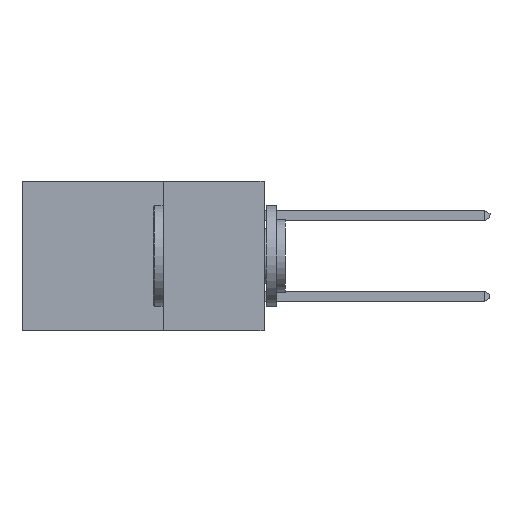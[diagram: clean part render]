
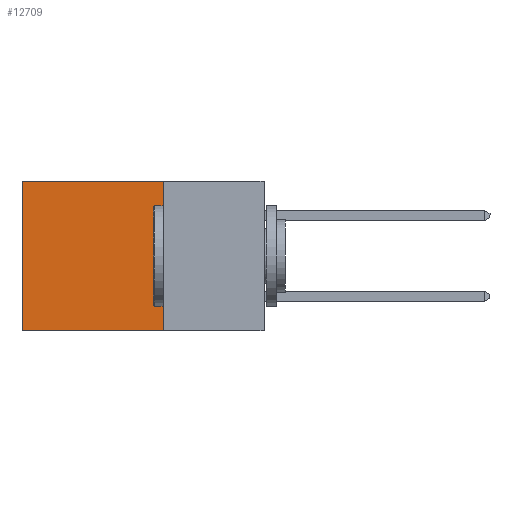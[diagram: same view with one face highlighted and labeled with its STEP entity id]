
A CAD part, left-side view. The second image highlights one B-rep face of the part: STEP entity #12709.
In plain terms, the highlighted planar face has unit normal (-1, 0, 0).
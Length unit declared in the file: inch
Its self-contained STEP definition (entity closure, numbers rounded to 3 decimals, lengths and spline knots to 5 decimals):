
#444 = DIRECTION ( 'NONE',  ( 0., 1., 0. ) ) ;
#577 = ORIENTED_EDGE ( 'NONE', *, *, #9181, .T. ) ;
#768 = VERTEX_POINT ( 'NONE', #5218 ) ;
#2378 = AXIS2_PLACEMENT_3D ( 'NONE', #11979, #4411, #13243 ) ;
#2916 = LINE ( 'NONE', #13124, #12667 ) ;
#3073 = PLANE ( 'NONE',  #2378 ) ;
#4386 = VECTOR ( 'NONE', #13675, 39.37008 ) ;
#4411 = DIRECTION ( 'NONE',  ( 1., 0., 0. ) ) ;
#4799 = LINE ( 'NONE', #8060, #4386 ) ;
#4808 = EDGE_CURVE ( 'NONE', #10295, #5547, #4799, .T. ) ;
#5218 = CARTESIAN_POINT ( 'NONE',  ( 0.298, 0.6, -0.37 ) ) ;
#5322 = DIRECTION ( 'NONE',  ( 0., 0., -1. ) ) ;
#5547 = VERTEX_POINT ( 'NONE', #6333 ) ;
#5662 = LINE ( 'NONE', #11592, #8214 ) ;
#6092 = VECTOR ( 'NONE', #10987, 39.37008 ) ;
#6333 = CARTESIAN_POINT ( 'NONE',  ( 0.298, 0.25, -0.37 ) ) ;
#7376 = ORIENTED_EDGE ( 'NONE', *, *, #13450, .F. ) ;
#7650 = ORIENTED_EDGE ( 'NONE', *, *, #10622, .T. ) ;
#7759 = ORIENTED_EDGE ( 'NONE', *, *, #4808, .F. ) ;
#8060 = CARTESIAN_POINT ( 'NONE',  ( 0.298, 0.25, 0. ) ) ;
#8214 = VECTOR ( 'NONE', #5322, 39.37008 ) ;
#9181 = EDGE_CURVE ( 'NONE', #10295, #11585, #9433, .T. ) ;
#9433 = LINE ( 'NONE', #14702, #6092 ) ;
#10295 = VERTEX_POINT ( 'NONE', #15718 ) ;
#10622 = EDGE_CURVE ( 'NONE', #11585, #768, #5662, .T. ) ;
#10961 = CARTESIAN_POINT ( 'NONE',  ( 0.298, 0.6, 0. ) ) ;
#10987 = DIRECTION ( 'NONE',  ( 0., 1., 0. ) ) ;
#11585 = VERTEX_POINT ( 'NONE', #10961 ) ;
#11592 = CARTESIAN_POINT ( 'NONE',  ( 0.298, 0.6, 0. ) ) ;
#11979 = CARTESIAN_POINT ( 'NONE',  ( 0.298, 0.25, 0. ) ) ;
#12667 = VECTOR ( 'NONE', #444, 39.37008 ) ;
#12709 = ADVANCED_FACE ( 'NONE', ( #14834 ), #3073, .F. ) ;
#13124 = CARTESIAN_POINT ( 'NONE',  ( 0.298, 0.25, -0.37 ) ) ;
#13243 = DIRECTION ( 'NONE',  ( 0., 0., -1. ) ) ;
#13450 = EDGE_CURVE ( 'NONE', #5547, #768, #2916, .T. ) ;
#13675 = DIRECTION ( 'NONE',  ( 0., 0., -1. ) ) ;
#14567 = EDGE_LOOP ( 'NONE', ( #7650, #7376, #7759, #577 ) ) ;
#14702 = CARTESIAN_POINT ( 'NONE',  ( 0.298, 0.25, 0. ) ) ;
#14834 = FACE_OUTER_BOUND ( 'NONE', #14567, .T. ) ;
#15718 = CARTESIAN_POINT ( 'NONE',  ( 0.298, 0.25, 0. ) ) ;
